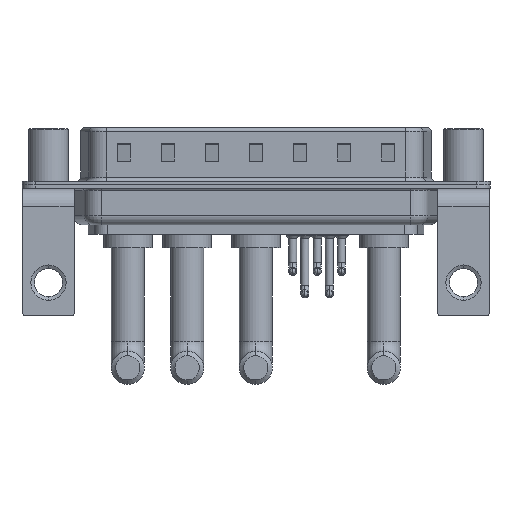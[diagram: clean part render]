
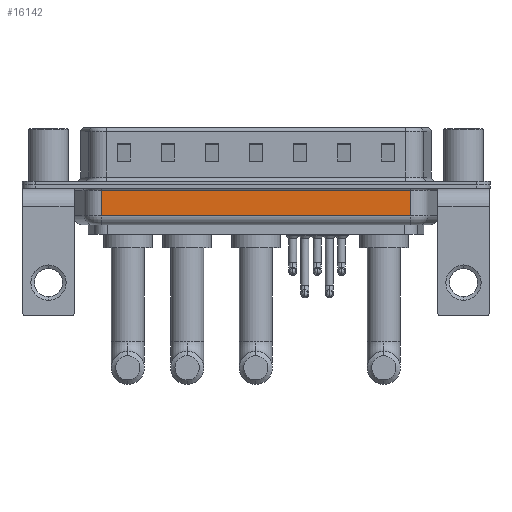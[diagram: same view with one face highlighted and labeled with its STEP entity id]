
A CAD part, front view. The second image highlights one B-rep face of the part: STEP entity #16142.
In plain terms, the highlighted planar face has unit normal (0, -1, 0).
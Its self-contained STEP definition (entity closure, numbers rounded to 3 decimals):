
#428 = CARTESIAN_POINT ( 'NONE',  ( 6.006, -5.35, -4.5 ) ) ;
#473 = EDGE_CURVE ( 'NONE', #2236, #11376, #1896, .T. ) ;
#1896 = LINE ( 'NONE', #13533, #6018 ) ;
#1948 = PLANE ( 'NONE',  #16694 ) ;
#2204 = FACE_OUTER_BOUND ( 'NONE', #7211, .T. ) ;
#2236 = VERTEX_POINT ( 'NONE', #22107 ) ;
#4005 = VERTEX_POINT ( 'NONE', #13512 ) ;
#4754 = VECTOR ( 'NONE', #18360, 1000. ) ;
#4919 = CARTESIAN_POINT ( 'NONE',  ( 6.006, -5.35, -4.5 ) ) ;
#5569 = LINE ( 'NONE', #7743, #19496 ) ;
#5885 = EDGE_CURVE ( 'NONE', #23183, #2236, #21911, .T. ) ;
#5980 = DIRECTION ( 'NONE',  ( 0., 0., 1. ) ) ;
#6018 = VECTOR ( 'NONE', #15036, 1000. ) ;
#6402 = CARTESIAN_POINT ( 'NONE',  ( 6.006, -5.35, -0.65 ) ) ;
#6502 = CARTESIAN_POINT ( 'NONE',  ( 41.044, -5.35, -4.5 ) ) ;
#7211 = EDGE_LOOP ( 'NONE', ( #15952, #23476, #24311, #24177 ) ) ;
#7229 = CARTESIAN_POINT ( 'NONE',  ( 41.044, -5.35, -3.5 ) ) ;
#7743 = CARTESIAN_POINT ( 'NONE',  ( 6.006, -5.35, -3.5 ) ) ;
#8301 = EDGE_CURVE ( 'NONE', #4005, #11376, #24128, .T. ) ;
#11376 = VERTEX_POINT ( 'NONE', #6402 ) ;
#13512 = CARTESIAN_POINT ( 'NONE',  ( 6.006, -5.35, -3.5 ) ) ;
#13533 = CARTESIAN_POINT ( 'NONE',  ( 6.006, -5.35, -0.65 ) ) ;
#15036 = DIRECTION ( 'NONE',  ( -1., 0., 0. ) ) ;
#15952 = ORIENTED_EDGE ( 'NONE', *, *, #8301, .F. ) ;
#16142 = ADVANCED_FACE ( 'NONE', ( #2204 ), #1948, .F. ) ;
#16371 = DIRECTION ( 'NONE',  ( 0., 0., 1. ) ) ;
#16694 = AXIS2_PLACEMENT_3D ( 'NONE', #428, #19638, #5980 ) ;
#18360 = DIRECTION ( 'NONE',  ( 0., 0., 1. ) ) ;
#18867 = DIRECTION ( 'NONE',  ( 1., 0., 0. ) ) ;
#19496 = VECTOR ( 'NONE', #18867, 1000. ) ;
#19638 = DIRECTION ( 'NONE',  ( 0., 1., 0. ) ) ;
#21911 = LINE ( 'NONE', #6502, #21961 ) ;
#21961 = VECTOR ( 'NONE', #16371, 1000. ) ;
#22107 = CARTESIAN_POINT ( 'NONE',  ( 41.044, -5.35, -0.65 ) ) ;
#23183 = VERTEX_POINT ( 'NONE', #7229 ) ;
#23476 = ORIENTED_EDGE ( 'NONE', *, *, #24554, .T. ) ;
#24128 = LINE ( 'NONE', #4919, #4754 ) ;
#24177 = ORIENTED_EDGE ( 'NONE', *, *, #473, .T. ) ;
#24311 = ORIENTED_EDGE ( 'NONE', *, *, #5885, .T. ) ;
#24554 = EDGE_CURVE ( 'NONE', #4005, #23183, #5569, .T. ) ;
